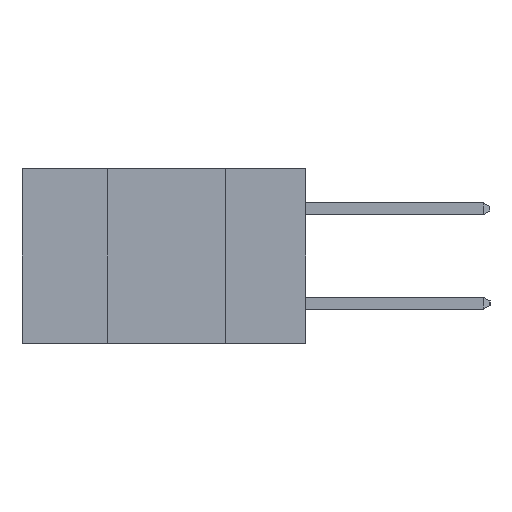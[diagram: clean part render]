
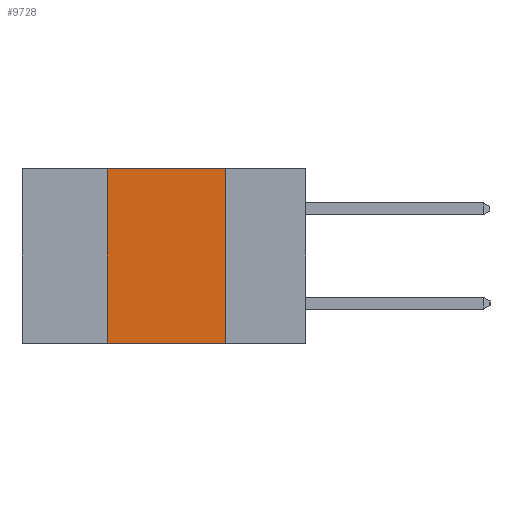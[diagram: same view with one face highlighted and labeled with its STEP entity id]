
A CAD part, left-side view. The second image highlights one B-rep face of the part: STEP entity #9728.
In plain terms, the highlighted planar face has unit normal (-1, 0, 0).
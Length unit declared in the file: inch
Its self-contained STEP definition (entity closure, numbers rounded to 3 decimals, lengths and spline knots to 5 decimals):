
#9 = CARTESIAN_POINT ( 'NONE',  ( 0., 0.42, -0.37 ) ) ;
#292 = VERTEX_POINT ( 'NONE', #13707 ) ;
#342 = DIRECTION ( 'NONE',  ( 0., -1., 0. ) ) ;
#810 = VERTEX_POINT ( 'NONE', #1404 ) ;
#911 = DIRECTION ( 'NONE',  ( 1., 0., 0. ) ) ;
#1105 = EDGE_CURVE ( 'NONE', #810, #292, #4732, .T. ) ;
#1404 = CARTESIAN_POINT ( 'NONE',  ( 0., 0.42, 0. ) ) ;
#1742 = EDGE_CURVE ( 'NONE', #7229, #9282, #11254, .T. ) ;
#1774 = ORIENTED_EDGE ( 'NONE', *, *, #13814, .F. ) ;
#3190 = LINE ( 'NONE', #12010, #4132 ) ;
#3331 = DIRECTION ( 'NONE',  ( 0., 0., 1. ) ) ;
#3840 = PLANE ( 'NONE',  #7612 ) ;
#4010 = VECTOR ( 'NONE', #342, 39.37008 ) ;
#4132 = VECTOR ( 'NONE', #3331, 39.37008 ) ;
#4436 = CARTESIAN_POINT ( 'NONE',  ( 0., 0.17, -0.37 ) ) ;
#4732 = LINE ( 'NONE', #9667, #9008 ) ;
#5684 = CARTESIAN_POINT ( 'NONE',  ( 0., 0.17, -0.37 ) ) ;
#6423 = FACE_OUTER_BOUND ( 'NONE', #11961, .T. ) ;
#7156 = DIRECTION ( 'NONE',  ( 0., 0., -1. ) ) ;
#7229 = VERTEX_POINT ( 'NONE', #9 ) ;
#7612 = AXIS2_PLACEMENT_3D ( 'NONE', #8214, #911, #11118 ) ;
#8214 = CARTESIAN_POINT ( 'NONE',  ( 0., 0.6, 0. ) ) ;
#8533 = VECTOR ( 'NONE', #7156, 39.37008 ) ;
#8826 = ORIENTED_EDGE ( 'NONE', *, *, #9460, .F. ) ;
#9008 = VECTOR ( 'NONE', #9549, 39.37008 ) ;
#9282 = VERTEX_POINT ( 'NONE', #4436 ) ;
#9460 = EDGE_CURVE ( 'NONE', #7229, #810, #3190, .T. ) ;
#9549 = DIRECTION ( 'NONE',  ( 0., -1., 0. ) ) ;
#9667 = CARTESIAN_POINT ( 'NONE',  ( 0., 0.6, 0. ) ) ;
#9728 = ADVANCED_FACE ( 'NONE', ( #6423 ), #3840, .F. ) ;
#11118 = DIRECTION ( 'NONE',  ( 0., 0., -1. ) ) ;
#11254 = LINE ( 'NONE', #18468, #4010 ) ;
#11804 = ORIENTED_EDGE ( 'NONE', *, *, #1105, .F. ) ;
#11961 = EDGE_LOOP ( 'NONE', ( #1774, #11804, #8826, #13504 ) ) ;
#12010 = CARTESIAN_POINT ( 'NONE',  ( 0., 0.42, -0.37 ) ) ;
#12377 = LINE ( 'NONE', #5684, #8533 ) ;
#13504 = ORIENTED_EDGE ( 'NONE', *, *, #1742, .T. ) ;
#13707 = CARTESIAN_POINT ( 'NONE',  ( 0., 0.17, 0. ) ) ;
#13814 = EDGE_CURVE ( 'NONE', #292, #9282, #12377, .T. ) ;
#18468 = CARTESIAN_POINT ( 'NONE',  ( 0., 0.6, -0.37 ) ) ;
